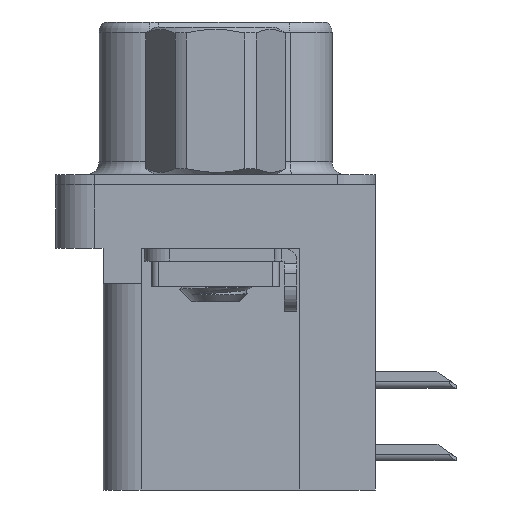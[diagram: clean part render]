
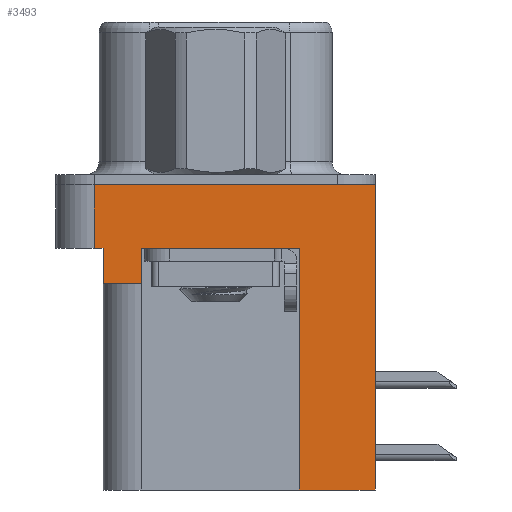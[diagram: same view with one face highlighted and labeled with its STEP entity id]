
A CAD part, left-side view. The second image highlights one B-rep face of the part: STEP entity #3493.
In plain terms, the highlighted planar face has unit normal (-1, 0, 0).
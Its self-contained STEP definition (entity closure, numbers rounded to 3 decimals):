
#399 = CARTESIAN_POINT ( 'NONE',  ( -2.935, 4.425, -2.5 ) ) ;
#824 = DIRECTION ( 'NONE',  ( 0., 0., 1. ) ) ;
#860 = DIRECTION ( 'NONE',  ( -1., 0., 0. ) ) ;
#1012 = CARTESIAN_POINT ( 'NONE',  ( -2.935, -6.275, -2.5 ) ) ;
#1277 = ORIENTED_EDGE ( 'NONE', *, *, #17881, .F. ) ;
#1457 = DIRECTION ( 'NONE',  ( 0., -1., 0. ) ) ;
#1510 = VERTEX_POINT ( 'NONE', #18535 ) ;
#2061 = CARTESIAN_POINT ( 'NONE',  ( -2.935, -6.275, 0. ) ) ;
#2157 = CARTESIAN_POINT ( 'NONE',  ( -2.935, 4.775, -2.5 ) ) ;
#3460 = CARTESIAN_POINT ( 'NONE',  ( -2.935, -6.275, -2.5 ) ) ;
#3493 = ADVANCED_FACE ( 'NONE', ( #7136 ), #4738, .T. ) ;
#3946 = ORIENTED_EDGE ( 'NONE', *, *, #17200, .F. ) ;
#4158 = DIRECTION ( 'NONE',  ( 0., 0., 1. ) ) ;
#4438 = CARTESIAN_POINT ( 'NONE',  ( -2.935, 4.425, -3.9 ) ) ;
#4589 = VERTEX_POINT ( 'NONE', #12092 ) ;
#4738 = PLANE ( 'NONE',  #7618 ) ;
#5147 = CARTESIAN_POINT ( 'NONE',  ( -2.935, 2.895, -2.5 ) ) ;
#5436 = DIRECTION ( 'NONE',  ( 0., 0., 1. ) ) ;
#5441 = EDGE_LOOP ( 'NONE', ( #17166, #22826, #9766, #15883, #3946, #20174, #11404, #1277, #11348, #12815 ) ) ;
#5618 = VECTOR ( 'NONE', #4158, 1000. ) ;
#5729 = LINE ( 'NONE', #10765, #6176 ) ;
#5826 = LINE ( 'NONE', #19629, #5618 ) ;
#6057 = VECTOR ( 'NONE', #8548, 1000. ) ;
#6155 = LINE ( 'NONE', #17681, #6057 ) ;
#6176 = VECTOR ( 'NONE', #23039, 1000. ) ;
#6207 = VECTOR ( 'NONE', #17549, 1000. ) ;
#6377 = LINE ( 'NONE', #14222, #6207 ) ;
#6830 = VECTOR ( 'NONE', #13936, 1000. ) ;
#6951 = VECTOR ( 'NONE', #8054, 1000. ) ;
#6964 = LINE ( 'NONE', #2061, #6951 ) ;
#6990 = LINE ( 'NONE', #2157, #6830 ) ;
#7136 = FACE_OUTER_BOUND ( 'NONE', #5441, .T. ) ;
#7410 = VERTEX_POINT ( 'NONE', #4438 ) ;
#7618 = AXIS2_PLACEMENT_3D ( 'NONE', #1012, #860, #824 ) ;
#7728 = VECTOR ( 'NONE', #21954, 1000. ) ;
#7985 = VERTEX_POINT ( 'NONE', #10034 ) ;
#7986 = VERTEX_POINT ( 'NONE', #399 ) ;
#8021 = LINE ( 'NONE', #3460, #7728 ) ;
#8054 = DIRECTION ( 'NONE',  ( 0., -1., 0. ) ) ;
#8548 = DIRECTION ( 'NONE',  ( 0., 0., 1. ) ) ;
#8662 = CARTESIAN_POINT ( 'NONE',  ( -2.935, 4.425, -3.9 ) ) ;
#8921 = VECTOR ( 'NONE', #21353, 1000. ) ;
#9161 = LINE ( 'NONE', #8662, #8921 ) ;
#9766 = ORIENTED_EDGE ( 'NONE', *, *, #17508, .T. ) ;
#10034 = CARTESIAN_POINT ( 'NONE',  ( -2.935, 2.895, -3.9 ) ) ;
#10368 = VERTEX_POINT ( 'NONE', #22996 ) ;
#10564 = VECTOR ( 'NONE', #5436, 1000. ) ;
#10765 = CARTESIAN_POINT ( 'NONE',  ( -2.935, -3.295, -12. ) ) ;
#11013 = LINE ( 'NONE', #18468, #10564 ) ;
#11348 = ORIENTED_EDGE ( 'NONE', *, *, #17915, .F. ) ;
#11403 = CARTESIAN_POINT ( 'NONE',  ( -2.935, -6.275, -2.5 ) ) ;
#11404 = ORIENTED_EDGE ( 'NONE', *, *, #11919, .T. ) ;
#11828 = VERTEX_POINT ( 'NONE', #5147 ) ;
#11919 = EDGE_CURVE ( 'NONE', #11828, #22931, #23710, .T. ) ;
#12092 = CARTESIAN_POINT ( 'NONE',  ( -2.935, 4.775, 0. ) ) ;
#12482 = CARTESIAN_POINT ( 'NONE',  ( -2.935, -3.295, -2.5 ) ) ;
#12815 = ORIENTED_EDGE ( 'NONE', *, *, #17947, .T. ) ;
#13414 = CARTESIAN_POINT ( 'NONE',  ( -2.935, -3.295, -12. ) ) ;
#13442 = EDGE_CURVE ( 'NONE', #7985, #11828, #11013, .T. ) ;
#13936 = DIRECTION ( 'NONE',  ( 0., 0., 1. ) ) ;
#14222 = CARTESIAN_POINT ( 'NONE',  ( -2.935, 4.425, -3.9 ) ) ;
#15883 = ORIENTED_EDGE ( 'NONE', *, *, #17860, .F. ) ;
#17166 = ORIENTED_EDGE ( 'NONE', *, *, #17725, .F. ) ;
#17200 = EDGE_CURVE ( 'NONE', #7985, #7410, #9161, .T. ) ;
#17508 = EDGE_CURVE ( 'NONE', #19100, #7986, #8021, .T. ) ;
#17549 = DIRECTION ( 'NONE',  ( 0., 0., 1. ) ) ;
#17681 = CARTESIAN_POINT ( 'NONE',  ( -2.935, -3.295, -12. ) ) ;
#17725 = EDGE_CURVE ( 'NONE', #4589, #1510, #6964, .T. ) ;
#17753 = EDGE_CURVE ( 'NONE', #19100, #4589, #6990, .T. ) ;
#17860 = EDGE_CURVE ( 'NONE', #7410, #7986, #6377, .T. ) ;
#17881 = EDGE_CURVE ( 'NONE', #19047, #22931, #6155, .T. ) ;
#17915 = EDGE_CURVE ( 'NONE', #10368, #19047, #5729, .T. ) ;
#17947 = EDGE_CURVE ( 'NONE', #10368, #1510, #5826, .T. ) ;
#18468 = CARTESIAN_POINT ( 'NONE',  ( -2.935, 2.895, -3.9 ) ) ;
#18535 = CARTESIAN_POINT ( 'NONE',  ( -2.935, -6.275, 0. ) ) ;
#19047 = VERTEX_POINT ( 'NONE', #13414 ) ;
#19100 = VERTEX_POINT ( 'NONE', #22207 ) ;
#19629 = CARTESIAN_POINT ( 'NONE',  ( -2.935, -6.275, -2.5 ) ) ;
#20174 = ORIENTED_EDGE ( 'NONE', *, *, #13442, .T. ) ;
#21353 = DIRECTION ( 'NONE',  ( 0., 1., 0. ) ) ;
#21954 = DIRECTION ( 'NONE',  ( 0., -1., 0. ) ) ;
#22207 = CARTESIAN_POINT ( 'NONE',  ( -2.935, 4.775, -2.5 ) ) ;
#22826 = ORIENTED_EDGE ( 'NONE', *, *, #17753, .F. ) ;
#22931 = VERTEX_POINT ( 'NONE', #12482 ) ;
#22996 = CARTESIAN_POINT ( 'NONE',  ( -2.935, -6.275, -12. ) ) ;
#23039 = DIRECTION ( 'NONE',  ( 0., 1., 0. ) ) ;
#23616 = VECTOR ( 'NONE', #1457, 1000. ) ;
#23710 = LINE ( 'NONE', #11403, #23616 ) ;
